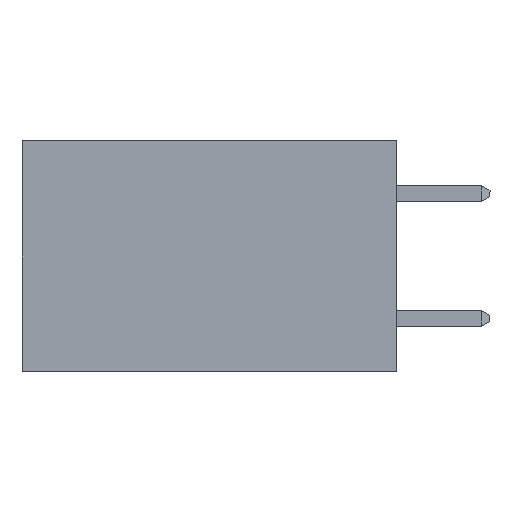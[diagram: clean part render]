
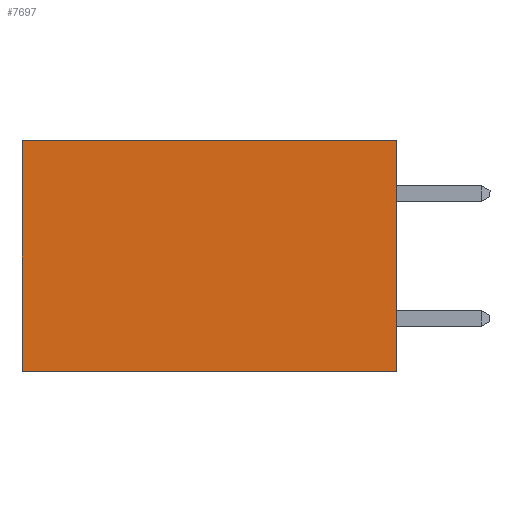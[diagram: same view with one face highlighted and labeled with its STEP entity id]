
A CAD part, left-side view. The second image highlights one B-rep face of the part: STEP entity #7697.
In plain terms, the highlighted planar face has unit normal (-1, 0, 0).
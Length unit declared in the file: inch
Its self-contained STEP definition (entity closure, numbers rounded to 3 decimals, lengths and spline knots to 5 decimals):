
#577 = CARTESIAN_POINT ( 'NONE',  ( 0.2615, 0., -0.37 ) ) ;
#749 = DIRECTION ( 'NONE',  ( 0., 0., -1. ) ) ;
#1064 = VECTOR ( 'NONE', #5562, 39.37008 ) ;
#1526 = DIRECTION ( 'NONE',  ( 0., 1., 0. ) ) ;
#1565 = LINE ( 'NONE', #3552, #2669 ) ;
#1723 = VECTOR ( 'NONE', #6550, 39.37008 ) ;
#2061 = CARTESIAN_POINT ( 'NONE',  ( 0.2615, 0., 0. ) ) ;
#2268 = CARTESIAN_POINT ( 'NONE',  ( 0.2615, 0.6, -0.37 ) ) ;
#2565 = CARTESIAN_POINT ( 'NONE',  ( 0.2615, 0., -0.37 ) ) ;
#2669 = VECTOR ( 'NONE', #1526, 39.37008 ) ;
#2906 = LINE ( 'NONE', #2268, #3863 ) ;
#3038 = EDGE_CURVE ( 'NONE', #5495, #4487, #2906, .T. ) ;
#3179 = CARTESIAN_POINT ( 'NONE',  ( 0.2615, 0., -0.37 ) ) ;
#3347 = CARTESIAN_POINT ( 'NONE',  ( 0.2615, 0., 0. ) ) ;
#3449 = EDGE_CURVE ( 'NONE', #6349, #5495, #5986, .T. ) ;
#3552 = CARTESIAN_POINT ( 'NONE',  ( 0.2615, 0., -0.37 ) ) ;
#3581 = DIRECTION ( 'NONE',  ( 0., 0., -1. ) ) ;
#3824 = VERTEX_POINT ( 'NONE', #2565 ) ;
#3863 = VECTOR ( 'NONE', #3581, 39.37008 ) ;
#3913 = EDGE_CURVE ( 'NONE', #6349, #3824, #8176, .T. ) ;
#3961 = DIRECTION ( 'NONE',  ( 1., 0., 0. ) ) ;
#4019 = ORIENTED_EDGE ( 'NONE', *, *, #3913, .F. ) ;
#4382 = EDGE_CURVE ( 'NONE', #3824, #4487, #1565, .T. ) ;
#4487 = VERTEX_POINT ( 'NONE', #6634 ) ;
#5125 = CARTESIAN_POINT ( 'NONE',  ( 0.2615, 0.6, 0. ) ) ;
#5495 = VERTEX_POINT ( 'NONE', #5125 ) ;
#5562 = DIRECTION ( 'NONE',  ( 0., 0., -1. ) ) ;
#5649 = AXIS2_PLACEMENT_3D ( 'NONE', #577, #3961, #749 ) ;
#5986 = LINE ( 'NONE', #2061, #1723 ) ;
#6058 = EDGE_LOOP ( 'NONE', ( #7038, #6079, #4019, #7413 ) ) ;
#6079 = ORIENTED_EDGE ( 'NONE', *, *, #4382, .F. ) ;
#6349 = VERTEX_POINT ( 'NONE', #3347 ) ;
#6428 = PLANE ( 'NONE',  #5649 ) ;
#6550 = DIRECTION ( 'NONE',  ( 0., 1., 0. ) ) ;
#6634 = CARTESIAN_POINT ( 'NONE',  ( 0.2615, 0.6, -0.37 ) ) ;
#7038 = ORIENTED_EDGE ( 'NONE', *, *, #3038, .T. ) ;
#7413 = ORIENTED_EDGE ( 'NONE', *, *, #3449, .T. ) ;
#7697 = ADVANCED_FACE ( 'NONE', ( #7764 ), #6428, .F. ) ;
#7764 = FACE_OUTER_BOUND ( 'NONE', #6058, .T. ) ;
#8176 = LINE ( 'NONE', #3179, #1064 ) ;
